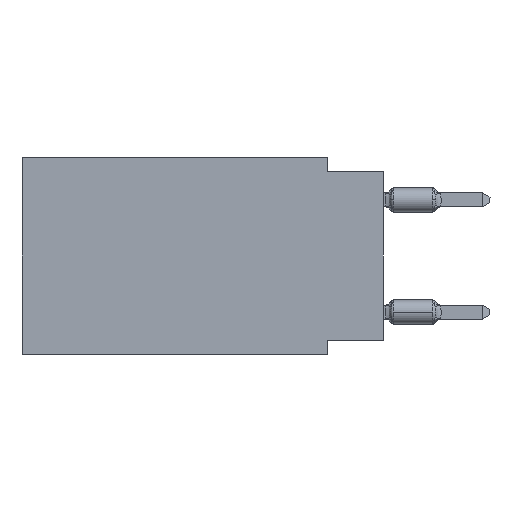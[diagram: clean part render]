
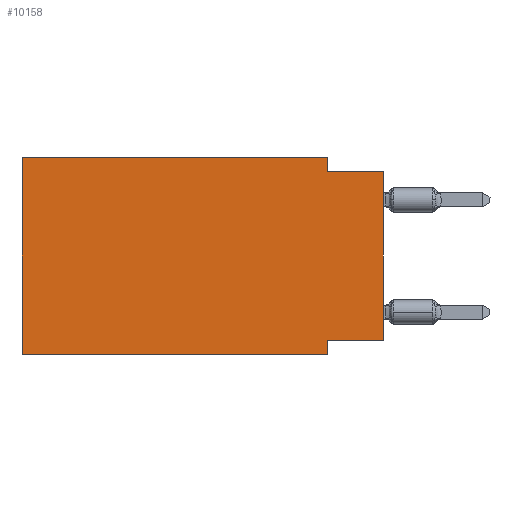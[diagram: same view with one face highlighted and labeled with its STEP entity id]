
A CAD part, left-side view. The second image highlights one B-rep face of the part: STEP entity #10158.
In plain terms, the highlighted planar face has unit normal (-1, 0, 0).
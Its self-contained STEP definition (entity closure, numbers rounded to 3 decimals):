
#50 = ORIENTED_EDGE ( 'NONE', *, *, #20619, .F. ) ;
#2092 = VERTEX_POINT ( 'NONE', #20101 ) ;
#2250 = LINE ( 'NONE', #13570, #20949 ) ;
#2814 = EDGE_CURVE ( 'NONE', #23096, #4313, #12790, .T. ) ;
#2905 = VERTEX_POINT ( 'NONE', #14160 ) ;
#3031 = DIRECTION ( 'NONE',  ( 0., 0., 1. ) ) ;
#3162 = VECTOR ( 'NONE', #18989, 1000. ) ;
#3198 = VERTEX_POINT ( 'NONE', #5225 ) ;
#3577 = CARTESIAN_POINT ( 'NONE',  ( 0., 2.54, 0. ) ) ;
#3944 = ORIENTED_EDGE ( 'NONE', *, *, #8360, .F. ) ;
#4118 = EDGE_CURVE ( 'NONE', #2092, #10318, #18082, .T. ) ;
#4164 = PLANE ( 'NONE',  #22315 ) ;
#4313 = VERTEX_POINT ( 'NONE', #17819 ) ;
#4464 = CARTESIAN_POINT ( 'NONE',  ( 0., 0., -8.255 ) ) ;
#4909 = LINE ( 'NONE', #10447, #21873 ) ;
#5062 = DIRECTION ( 'NONE',  ( 0., 0., -1. ) ) ;
#5225 = CARTESIAN_POINT ( 'NONE',  ( 0., 0., -0.635 ) ) ;
#5960 = EDGE_LOOP ( 'NONE', ( #10651, #3944, #9248, #18399, #50, #6770, #23570, #17413 ) ) ;
#6249 = DIRECTION ( 'NONE',  ( 1., 0., 0. ) ) ;
#6489 = DIRECTION ( 'NONE',  ( 0., 0., -1. ) ) ;
#6770 = ORIENTED_EDGE ( 'NONE', *, *, #2814, .T. ) ;
#6845 = CARTESIAN_POINT ( 'NONE',  ( 0., 2.54, 0. ) ) ;
#7842 = FACE_OUTER_BOUND ( 'NONE', #5960, .T. ) ;
#8360 = EDGE_CURVE ( 'NONE', #16615, #3198, #15905, .T. ) ;
#8975 = LINE ( 'NONE', #3577, #21979 ) ;
#9248 = ORIENTED_EDGE ( 'NONE', *, *, #24059, .F. ) ;
#9619 = DIRECTION ( 'NONE',  ( 0., 0., -1. ) ) ;
#9759 = LINE ( 'NONE', #13460, #3162 ) ;
#9953 = VECTOR ( 'NONE', #18075, 1000. ) ;
#10158 = ADVANCED_FACE ( 'NONE', ( #7842 ), #4164, .F. ) ;
#10318 = VERTEX_POINT ( 'NONE', #6845 ) ;
#10410 = CARTESIAN_POINT ( 'NONE',  ( 0., 16.383, 0. ) ) ;
#10447 = CARTESIAN_POINT ( 'NONE',  ( 0., 0., -8.255 ) ) ;
#10651 = ORIENTED_EDGE ( 'NONE', *, *, #19346, .T. ) ;
#12430 = DIRECTION ( 'NONE',  ( 0., 1., 0. ) ) ;
#12440 = DIRECTION ( 'NONE',  ( 0., -1., 0. ) ) ;
#12462 = VECTOR ( 'NONE', #12440, 1000. ) ;
#12790 = LINE ( 'NONE', #18191, #9953 ) ;
#13460 = CARTESIAN_POINT ( 'NONE',  ( 0., 0., 0. ) ) ;
#13570 = CARTESIAN_POINT ( 'NONE',  ( 0., 2.54, -8.89 ) ) ;
#14160 = CARTESIAN_POINT ( 'NONE',  ( 0., 2.54, -8.255 ) ) ;
#14207 = EDGE_CURVE ( 'NONE', #22706, #2905, #4909, .T. ) ;
#14350 = LINE ( 'NONE', #10410, #16540 ) ;
#15664 = CARTESIAN_POINT ( 'NONE',  ( 0., 0., -0.635 ) ) ;
#15905 = LINE ( 'NONE', #15664, #23412 ) ;
#16343 = CARTESIAN_POINT ( 'NONE',  ( 0., 16.383, 0. ) ) ;
#16540 = VECTOR ( 'NONE', #3031, 1000. ) ;
#16615 = VERTEX_POINT ( 'NONE', #17526 ) ;
#16903 = EDGE_CURVE ( 'NONE', #2905, #4313, #2250, .T. ) ;
#17413 = ORIENTED_EDGE ( 'NONE', *, *, #14207, .F. ) ;
#17511 = DIRECTION ( 'NONE',  ( 0., -1., 0. ) ) ;
#17526 = CARTESIAN_POINT ( 'NONE',  ( 0., 2.54, -0.635 ) ) ;
#17819 = CARTESIAN_POINT ( 'NONE',  ( 0., 2.54, -8.89 ) ) ;
#18075 = DIRECTION ( 'NONE',  ( 0., -1., 0. ) ) ;
#18082 = LINE ( 'NONE', #16343, #12462 ) ;
#18191 = CARTESIAN_POINT ( 'NONE',  ( 0., 16.383, -8.89 ) ) ;
#18399 = ORIENTED_EDGE ( 'NONE', *, *, #4118, .F. ) ;
#18989 = DIRECTION ( 'NONE',  ( 0., 0., 1. ) ) ;
#19346 = EDGE_CURVE ( 'NONE', #22706, #3198, #9759, .T. ) ;
#19657 = CARTESIAN_POINT ( 'NONE',  ( 0., 16.383, 0. ) ) ;
#20101 = CARTESIAN_POINT ( 'NONE',  ( 0., 16.383, 0. ) ) ;
#20619 = EDGE_CURVE ( 'NONE', #23096, #2092, #14350, .T. ) ;
#20949 = VECTOR ( 'NONE', #9619, 1000. ) ;
#21873 = VECTOR ( 'NONE', #12430, 1000. ) ;
#21979 = VECTOR ( 'NONE', #5062, 1000. ) ;
#22315 = AXIS2_PLACEMENT_3D ( 'NONE', #19657, #6249, #6489 ) ;
#22706 = VERTEX_POINT ( 'NONE', #4464 ) ;
#23096 = VERTEX_POINT ( 'NONE', #23350 ) ;
#23350 = CARTESIAN_POINT ( 'NONE',  ( 0., 16.383, -8.89 ) ) ;
#23412 = VECTOR ( 'NONE', #17511, 1000. ) ;
#23570 = ORIENTED_EDGE ( 'NONE', *, *, #16903, .F. ) ;
#24059 = EDGE_CURVE ( 'NONE', #10318, #16615, #8975, .T. ) ;
